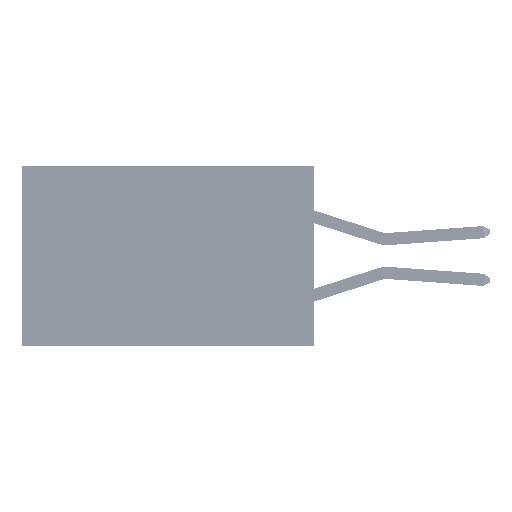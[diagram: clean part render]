
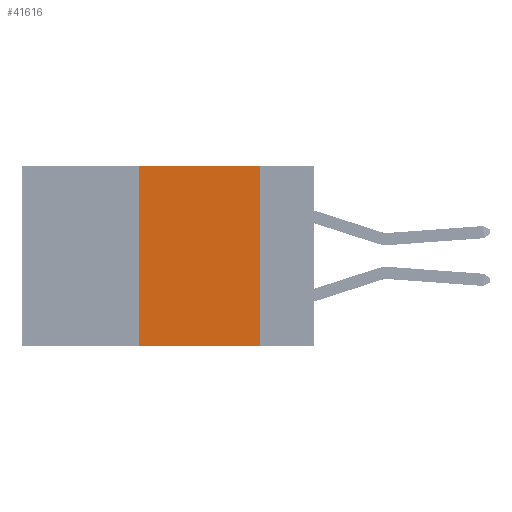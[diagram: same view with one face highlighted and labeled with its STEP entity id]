
A CAD part, left-side view. The second image highlights one B-rep face of the part: STEP entity #41616.
In plain terms, the highlighted planar face has unit normal (-1, 0, 0).
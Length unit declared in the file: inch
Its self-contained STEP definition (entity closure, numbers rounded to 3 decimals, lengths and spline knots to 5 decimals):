
#1557 = EDGE_CURVE ( 'NONE', #3950, #33416, #18374, .T. ) ;
#1739 = FACE_OUTER_BOUND ( 'NONE', #4502, .T. ) ;
#2746 = AXIS2_PLACEMENT_3D ( 'NONE', #32572, #45012, #4860 ) ;
#3950 = VERTEX_POINT ( 'NONE', #7485 ) ;
#4502 = EDGE_LOOP ( 'NONE', ( #31970, #34587, #25403, #26564 ) ) ;
#4860 = DIRECTION ( 'NONE',  ( 0., 0., -1. ) ) ;
#7377 = EDGE_CURVE ( 'NONE', #33416, #36399, #36511, .T. ) ;
#7485 = CARTESIAN_POINT ( 'NONE',  ( 0., 0.36, 0. ) ) ;
#9140 = VECTOR ( 'NONE', #38574, 39.37008 ) ;
#11494 = EDGE_CURVE ( 'NONE', #29404, #3950, #26663, .T. ) ;
#11772 = VECTOR ( 'NONE', #48446, 39.37008 ) ;
#11889 = CARTESIAN_POINT ( 'NONE',  ( 0., 0.11, -0.37 ) ) ;
#13973 = CARTESIAN_POINT ( 'NONE',  ( 0., 0.11, 0. ) ) ;
#15241 = DIRECTION ( 'NONE',  ( 0., -1., 0. ) ) ;
#17542 = PLANE ( 'NONE',  #2746 ) ;
#18374 = LINE ( 'NONE', #19124, #9140 ) ;
#19124 = CARTESIAN_POINT ( 'NONE',  ( 0., 0.6, 0. ) ) ;
#20407 = VECTOR ( 'NONE', #15241, 39.37008 ) ;
#22785 = CARTESIAN_POINT ( 'NONE',  ( 0., 0.36, 0. ) ) ;
#23005 = CARTESIAN_POINT ( 'NONE',  ( 0., 0.6, -0.37 ) ) ;
#25403 = ORIENTED_EDGE ( 'NONE', *, *, #11494, .F. ) ;
#26564 = ORIENTED_EDGE ( 'NONE', *, *, #30332, .T. ) ;
#26663 = LINE ( 'NONE', #22785, #37541 ) ;
#29404 = VERTEX_POINT ( 'NONE', #35299 ) ;
#30332 = EDGE_CURVE ( 'NONE', #29404, #36399, #45831, .T. ) ;
#31970 = ORIENTED_EDGE ( 'NONE', *, *, #7377, .F. ) ;
#32572 = CARTESIAN_POINT ( 'NONE',  ( 0., 0.6, 0. ) ) ;
#33416 = VERTEX_POINT ( 'NONE', #42652 ) ;
#34587 = ORIENTED_EDGE ( 'NONE', *, *, #1557, .F. ) ;
#35299 = CARTESIAN_POINT ( 'NONE',  ( 0., 0.36, -0.37 ) ) ;
#36399 = VERTEX_POINT ( 'NONE', #11889 ) ;
#36511 = LINE ( 'NONE', #13973, #11772 ) ;
#37541 = VECTOR ( 'NONE', #38592, 39.37008 ) ;
#38574 = DIRECTION ( 'NONE',  ( 0., -1., 0. ) ) ;
#38592 = DIRECTION ( 'NONE',  ( 0., 0., 1. ) ) ;
#41616 = ADVANCED_FACE ( 'NONE', ( #1739 ), #17542, .F. ) ;
#42652 = CARTESIAN_POINT ( 'NONE',  ( 0., 0.11, 0. ) ) ;
#45012 = DIRECTION ( 'NONE',  ( 1., 0., 0. ) ) ;
#45831 = LINE ( 'NONE', #23005, #20407 ) ;
#48446 = DIRECTION ( 'NONE',  ( 0., 0., -1. ) ) ;
